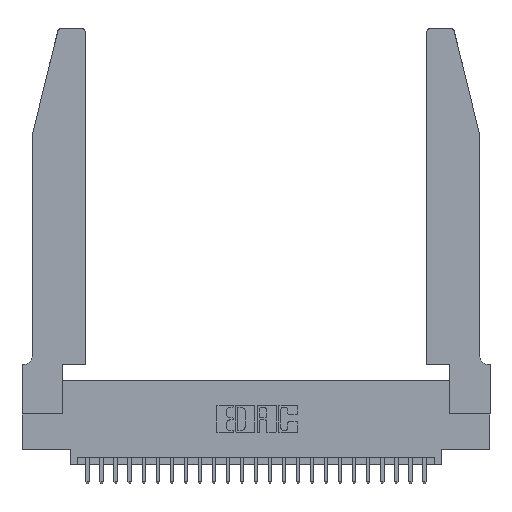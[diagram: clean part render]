
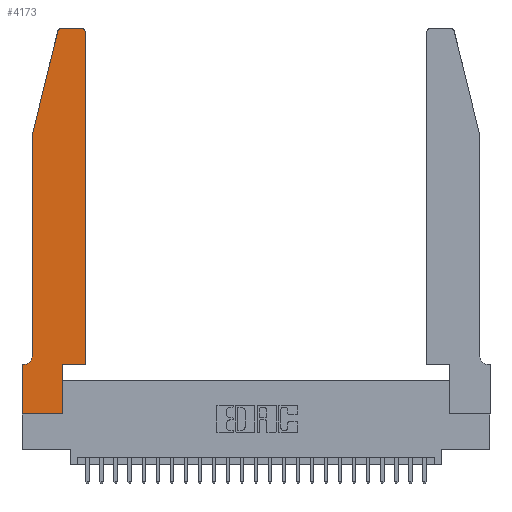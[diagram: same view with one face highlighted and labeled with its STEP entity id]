
A CAD part, top view. The second image highlights one B-rep face of the part: STEP entity #4173.
In plain terms, the highlighted planar face has unit normal (0, 0, 1).
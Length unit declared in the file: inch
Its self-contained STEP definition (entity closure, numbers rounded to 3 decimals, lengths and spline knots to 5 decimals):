
#164 = ORIENTED_EDGE ( 'NONE', *, *, #10140, .T. ) ;
#378 = PLANE ( 'NONE',  #11656 ) ;
#737 = LINE ( 'NONE', #1184, #11224 ) ;
#884 = CARTESIAN_POINT ( 'NONE',  ( 0.4505, 0.35, 0.37 ) ) ;
#1017 = EDGE_CURVE ( 'NONE', #21041, #17866, #7623, .T. ) ;
#1184 = CARTESIAN_POINT ( 'NONE',  ( 0.2865, 0.35, 0.37 ) ) ;
#1460 = DIRECTION ( 'NONE',  ( 1., 0., 0. ) ) ;
#1795 = CIRCLE ( 'NONE', #8783, 0.03 ) ;
#2000 = CARTESIAN_POINT ( 'NONE',  ( 0.284, 2.75, 0.37 ) ) ;
#2527 = DIRECTION ( 'NONE',  ( 1., 0., 0. ) ) ;
#2530 = VECTOR ( 'NONE', #26069, 39.37008 ) ;
#2628 = CARTESIAN_POINT ( 'NONE',  ( 0.0755, 2., 0.37 ) ) ;
#2777 = CARTESIAN_POINT ( 'NONE',  ( 0.4505, 0.35, 0.37 ) ) ;
#2881 = ORIENTED_EDGE ( 'NONE', *, *, #22260, .T. ) ;
#2894 = ORIENTED_EDGE ( 'NONE', *, *, #5183, .T. ) ;
#3076 = VECTOR ( 'NONE', #17627, 39.37008 ) ;
#3096 = CARTESIAN_POINT ( 'NONE',  ( 0., 0., 0.37 ) ) ;
#3654 = EDGE_CURVE ( 'NONE', #21711, #24128, #8125, .T. ) ;
#3873 = CARTESIAN_POINT ( 'NONE',  ( 0.2865, 0., 0.37 ) ) ;
#4058 = DIRECTION ( 'NONE',  ( -0.239, -0.971, 0. ) ) ;
#4089 = CARTESIAN_POINT ( 'NONE',  ( 0.0755, 2., 0.37 ) ) ;
#4173 = ADVANCED_FACE ( 'NONE', ( #19694 ), #378, .T. ) ;
#4562 = CARTESIAN_POINT ( 'NONE',  ( 0., 0.35, 0.37 ) ) ;
#4614 = VECTOR ( 'NONE', #11091, 39.37008 ) ;
#4846 = LINE ( 'NONE', #4089, #20679 ) ;
#5126 = CARTESIAN_POINT ( 'NONE',  ( 0.4505, 0.35, 0.37 ) ) ;
#5183 = EDGE_CURVE ( 'NONE', #17866, #20561, #1795, .T. ) ;
#5447 = EDGE_CURVE ( 'NONE', #20561, #24805, #13180, .T. ) ;
#5536 = DIRECTION ( 'NONE',  ( 0., 1., 0. ) ) ;
#5687 = CARTESIAN_POINT ( 'NONE',  ( 0., 0.35, 0.37 ) ) ;
#5908 = ORIENTED_EDGE ( 'NONE', *, *, #12219, .T. ) ;
#6335 = VECTOR ( 'NONE', #4058, 39.37008 ) ;
#6580 = DIRECTION ( 'NONE',  ( 0., 0., 1. ) ) ;
#6778 = VECTOR ( 'NONE', #7636, 39.37008 ) ;
#7623 = LINE ( 'NONE', #884, #18607 ) ;
#7636 = DIRECTION ( 'NONE',  ( -1., 0., 0. ) ) ;
#8125 = LINE ( 'NONE', #25972, #2530 ) ;
#8783 = AXIS2_PLACEMENT_3D ( 'NONE', #26199, #13933, #1460 ) ;
#9912 = CARTESIAN_POINT ( 'NONE',  ( 0.0055, 0.35, 0.37 ) ) ;
#9971 = CARTESIAN_POINT ( 'NONE',  ( 0.0055, 0.42, 0.37 ) ) ;
#10017 = EDGE_LOOP ( 'NONE', ( #19710, #2881, #21067, #164, #26779, #19411, #15890, #17850, #5908, #10779, #20735, #2894 ) ) ;
#10140 = EDGE_CURVE ( 'NONE', #26812, #18360, #4846, .T. ) ;
#10540 = EDGE_CURVE ( 'NONE', #14284, #20627, #18434, .T. ) ;
#10779 = ORIENTED_EDGE ( 'NONE', *, *, #14121, .T. ) ;
#11091 = DIRECTION ( 'NONE',  ( 1., 0., 0. ) ) ;
#11224 = VECTOR ( 'NONE', #5536, 39.37008 ) ;
#11656 = AXIS2_PLACEMENT_3D ( 'NONE', #4562, #14986, #2527 ) ;
#11774 = CARTESIAN_POINT ( 'NONE',  ( 0.2865, 0.35, 0.37 ) ) ;
#11867 = VECTOR ( 'NONE', #20769, 39.37008 ) ;
#12024 = DIRECTION ( 'NONE',  ( -1., 0., 0. ) ) ;
#12219 = EDGE_CURVE ( 'NONE', #24128, #23202, #737, .T. ) ;
#13180 = LINE ( 'NONE', #16642, #11867 ) ;
#13379 = DIRECTION ( 'NONE',  ( 0., 1., 0. ) ) ;
#13933 = DIRECTION ( 'NONE',  ( 0., 0., 1. ) ) ;
#14121 = EDGE_CURVE ( 'NONE', #23202, #21041, #26514, .T. ) ;
#14284 = VERTEX_POINT ( 'NONE', #9912 ) ;
#14892 = EDGE_CURVE ( 'NONE', #18360, #14284, #25524, .T. ) ;
#14986 = DIRECTION ( 'NONE',  ( 0., 0., 1. ) ) ;
#15890 = ORIENTED_EDGE ( 'NONE', *, *, #21865, .T. ) ;
#16642 = CARTESIAN_POINT ( 'NONE',  ( 0.2605, 2.75, 0.37 ) ) ;
#17104 = CARTESIAN_POINT ( 'NONE',  ( 0., 0., 0.37 ) ) ;
#17627 = DIRECTION ( 'NONE',  ( 0., -1., 0. ) ) ;
#17636 = AXIS2_PLACEMENT_3D ( 'NONE', #9971, #24336, #12024 ) ;
#17850 = ORIENTED_EDGE ( 'NONE', *, *, #3654, .T. ) ;
#17866 = VERTEX_POINT ( 'NONE', #26220 ) ;
#18360 = VERTEX_POINT ( 'NONE', #25222 ) ;
#18434 = LINE ( 'NONE', #21935, #6778 ) ;
#18607 = VECTOR ( 'NONE', #13379, 39.37008 ) ;
#18647 = CARTESIAN_POINT ( 'NONE',  ( 0.0755, 2., 0.37 ) ) ;
#18958 = CARTESIAN_POINT ( 'NONE',  ( 0.284, 2.72, 0.37 ) ) ;
#19411 = ORIENTED_EDGE ( 'NONE', *, *, #10540, .T. ) ;
#19694 = FACE_OUTER_BOUND ( 'NONE', #10017, .T. ) ;
#19710 = ORIENTED_EDGE ( 'NONE', *, *, #5447, .T. ) ;
#20513 = AXIS2_PLACEMENT_3D ( 'NONE', #18958, #6580, #21003 ) ;
#20561 = VERTEX_POINT ( 'NONE', #26004 ) ;
#20574 = CARTESIAN_POINT ( 'NONE',  ( 0.25487, 2.72718, 0.37 ) ) ;
#20627 = VERTEX_POINT ( 'NONE', #5687 ) ;
#20679 = VECTOR ( 'NONE', #26777, 39.37008 ) ;
#20735 = ORIENTED_EDGE ( 'NONE', *, *, #1017, .T. ) ;
#20769 = DIRECTION ( 'NONE',  ( -1., 0., 0. ) ) ;
#21003 = DIRECTION ( 'NONE',  ( 1., 0., 0. ) ) ;
#21041 = VERTEX_POINT ( 'NONE', #5126 ) ;
#21067 = ORIENTED_EDGE ( 'NONE', *, *, #23405, .T. ) ;
#21711 = VERTEX_POINT ( 'NONE', #17104 ) ;
#21865 = EDGE_CURVE ( 'NONE', #20627, #21711, #25042, .T. ) ;
#21935 = CARTESIAN_POINT ( 'NONE',  ( 0.0755, 0.35, 0.37 ) ) ;
#22144 = VERTEX_POINT ( 'NONE', #20574 ) ;
#22260 = EDGE_CURVE ( 'NONE', #24805, #22144, #26287, .T. ) ;
#23202 = VERTEX_POINT ( 'NONE', #11774 ) ;
#23405 = EDGE_CURVE ( 'NONE', #22144, #26812, #23422, .T. ) ;
#23422 = LINE ( 'NONE', #18647, #6335 ) ;
#24128 = VERTEX_POINT ( 'NONE', #3873 ) ;
#24336 = DIRECTION ( 'NONE',  ( 0., 0., -1. ) ) ;
#24805 = VERTEX_POINT ( 'NONE', #2000 ) ;
#25042 = LINE ( 'NONE', #3096, #3076 ) ;
#25222 = CARTESIAN_POINT ( 'NONE',  ( 0.0755, 0.42, 0.37 ) ) ;
#25524 = CIRCLE ( 'NONE', #17636, 0.07 ) ;
#25972 = CARTESIAN_POINT ( 'NONE',  ( 0., 0., 0.37 ) ) ;
#26004 = CARTESIAN_POINT ( 'NONE',  ( 0.4205, 2.75, 0.37 ) ) ;
#26069 = DIRECTION ( 'NONE',  ( 1., 0., 0. ) ) ;
#26199 = CARTESIAN_POINT ( 'NONE',  ( 0.4205, 2.72, 0.37 ) ) ;
#26220 = CARTESIAN_POINT ( 'NONE',  ( 0.4505, 2.72, 0.37 ) ) ;
#26287 = CIRCLE ( 'NONE', #20513, 0.03 ) ;
#26514 = LINE ( 'NONE', #2777, #4614 ) ;
#26777 = DIRECTION ( 'NONE',  ( 0., -1., 0. ) ) ;
#26779 = ORIENTED_EDGE ( 'NONE', *, *, #14892, .T. ) ;
#26812 = VERTEX_POINT ( 'NONE', #2628 ) ;
